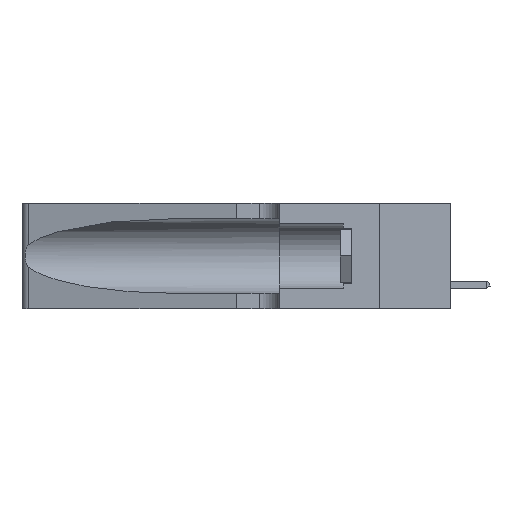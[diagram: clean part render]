
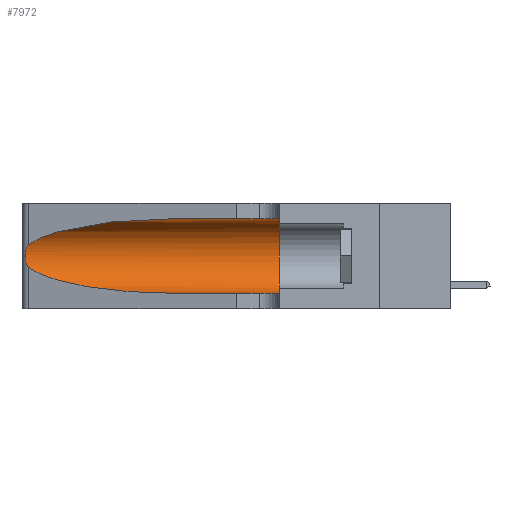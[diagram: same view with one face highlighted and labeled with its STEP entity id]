
A CAD part, left-side view. The second image highlights one B-rep face of the part: STEP entity #7972.
In plain terms, the highlighted cylindrical face has radius 3.308 mm (diameter 6.617 mm), a partial arc.
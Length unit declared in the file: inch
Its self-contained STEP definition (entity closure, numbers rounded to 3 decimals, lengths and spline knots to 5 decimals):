
#266 = CARTESIAN_POINT ( 'NONE',  ( 0.25555, 1.22993, 0.14849 ) ) ;
#973 = CARTESIAN_POINT ( 'NONE',  ( 0.1305, 0.72297, 0.05475 ) ) ;
#1196 = CARTESIAN_POINT ( 'NONE',  ( 0.25487, 1.22718, 0.14631 ) ) ;
#1910 = CARTESIAN_POINT ( 'NONE',  ( 0.1305, 0.35, 0.05475 ) ) ;
#3425 = CARTESIAN_POINT ( 'NONE',  ( 0.25555, 1.22994, 0.2215 ) ) ;
#3551 = CARTESIAN_POINT ( 'NONE',  ( 0.25487, 1.22718, 0.14631 ) ) ;
#4069 = DIRECTION ( 'NONE',  ( 0., 0., -1. ) ) ;
#4096 = EDGE_CURVE ( 'NONE', #28286, #34530, #33851, .T. ) ;
#5048 = VERTEX_POINT ( 'NONE', #1910 ) ;
#7972 = ADVANCED_FACE ( 'NONE', ( #28597 ), #37696, .F. ) ;
#8712 = CARTESIAN_POINT ( 'NONE',  ( 0.25487, 1.22718, 0.14631 ) ) ;
#9499 = ORIENTED_EDGE ( 'NONE', *, *, #19498, .T. ) ;
#9645 = CARTESIAN_POINT ( 'NONE',  ( 0.25487, 1.22718, 0.22369 ) ) ;
#9811 = CARTESIAN_POINT ( 'NONE',  ( 0.26018, 1.23835, 0.19895 ) ) ;
#9944 = CARTESIAN_POINT ( 'NONE',  ( 0.25639, 1.23184, 0.21858 ) ) ;
#10716 = CARTESIAN_POINT ( 'NONE',  ( 0.1305, 1.61858, 0.05475 ) ) ;
#10970 = VERTEX_POINT ( 'NONE', #23333 ) ;
#11529 = CARTESIAN_POINT ( 'NONE',  ( 0.1305, 0.72297, 0.05475 ) ) ;
#12513 = VERTEX_POINT ( 'NONE', #13545 ) ;
#13158 = CARTESIAN_POINT ( 'NONE',  ( 0.25789, 1.23486, 0.15765 ) ) ;
#13545 = CARTESIAN_POINT ( 'NONE',  ( 0.25487, 1.22718, 0.22369 ) ) ;
#16264 = CARTESIAN_POINT ( 'NONE',  ( 0.26075, 1.23896, 0.178 ) ) ;
#16585 = AXIS2_PLACEMENT_3D ( 'NONE', #17605, #33101, #27310 ) ;
#17440 = CARTESIAN_POINT ( 'NONE',  ( 0.2373, 1.15595, 0.08982 ) ) ;
#17605 = CARTESIAN_POINT ( 'NONE',  ( 0.1305, 0.35, 0.185 ) ) ;
#17712 = ORIENTED_EDGE ( 'NONE', *, *, #37765, .F. ) ;
#17723 = CARTESIAN_POINT ( 'NONE',  ( 0.18966, 0.96281, 0.05475 ) ) ;
#17938 = EDGE_LOOP ( 'NONE', ( #9499, #37967, #29278, #35419, #27481, #17712 ) ) ;
#19235 = CARTESIAN_POINT ( 'NONE',  ( 0.25854, 1.2359, 0.20912 ) ) ;
#19498 = EDGE_CURVE ( 'NONE', #28232, #12513, #19628, .T. ) ;
#19628 =( BOUNDED_CURVE ( )  B_SPLINE_CURVE ( 3, ( #27132, #28689, #23798, #9645 ),
 .UNSPECIFIED., .F., .F. ) 
 B_SPLINE_CURVE_WITH_KNOTS ( ( 4, 4 ),
 ( 1.5708, 2.84003 ),
 .UNSPECIFIED. ) 
 CURVE ( )  GEOMETRIC_REPRESENTATION_ITEM ( )  RATIONAL_B_SPLINE_CURVE ( ( 1., 0.87, 0.87, 1. ) ) 
 REPRESENTATION_ITEM ( '' )  );
#21260 = CARTESIAN_POINT ( 'NONE',  ( 0.1305, 0.72297, 0.31525 ) ) ;
#21829 = CIRCLE ( 'NONE', #16585, 0.13025 ) ;
#22750 = CARTESIAN_POINT ( 'NONE',  ( 0.25787, 1.23484, 0.2124 ) ) ;
#22917 = VECTOR ( 'NONE', #32781, 39.37008 ) ;
#23333 = CARTESIAN_POINT ( 'NONE',  ( 0.1305, 0.35, 0.31525 ) ) ;
#23798 = CARTESIAN_POINT ( 'NONE',  ( 0.2373, 1.15595, 0.28018 ) ) ;
#26509 = DIRECTION ( 'NONE',  ( 0., -1., 0. ) ) ;
#26532 = EDGE_CURVE ( 'NONE', #12513, #28286, #36415, .T. ) ;
#27076 = AXIS2_PLACEMENT_3D ( 'NONE', #28669, #26509, #4069 ) ;
#27132 = CARTESIAN_POINT ( 'NONE',  ( 0.1305, 0.72297, 0.31525 ) ) ;
#27310 = DIRECTION ( 'NONE',  ( 0., 0., 1. ) ) ;
#27481 = ORIENTED_EDGE ( 'NONE', *, *, #29092, .F. ) ;
#28232 = VERTEX_POINT ( 'NONE', #21260 ) ;
#28286 = VERTEX_POINT ( 'NONE', #8712 ) ;
#28597 = FACE_OUTER_BOUND ( 'NONE', #17938, .T. ) ;
#28669 = CARTESIAN_POINT ( 'NONE',  ( 0.1305, 1.61858, 0.185 ) ) ;
#28689 = CARTESIAN_POINT ( 'NONE',  ( 0.18966, 0.96281, 0.31525 ) ) ;
#28943 = CARTESIAN_POINT ( 'NONE',  ( 0.26075, 1.23896, 0.19203 ) ) ;
#29024 = VECTOR ( 'NONE', #39477, 39.37008 ) ;
#29092 = EDGE_CURVE ( 'NONE', #10970, #5048, #21829, .T. ) ;
#29209 = CARTESIAN_POINT ( 'NONE',  ( 0.26017, 1.23833, 0.17102 ) ) ;
#29278 = ORIENTED_EDGE ( 'NONE', *, *, #4096, .T. ) ;
#29430 = LINE ( 'NONE', #35769, #22917 ) ;
#32454 = CARTESIAN_POINT ( 'NONE',  ( 0.25856, 1.23593, 0.16098 ) ) ;
#32781 = DIRECTION ( 'NONE',  ( 0., -1., 0. ) ) ;
#33101 = DIRECTION ( 'NONE',  ( 0., 1., 0. ) ) ;
#33523 = LINE ( 'NONE', #10716, #29024 ) ;
#33851 =( BOUNDED_CURVE ( )  B_SPLINE_CURVE ( 3, ( #1196, #17440, #17723, #11529 ),
 .UNSPECIFIED., .F., .F. ) 
 B_SPLINE_CURVE_WITH_KNOTS ( ( 4, 4 ),
 ( 3.44316, 4.71239 ),
 .UNSPECIFIED. ) 
 CURVE ( )  GEOMETRIC_REPRESENTATION_ITEM ( )  RATIONAL_B_SPLINE_CURVE ( ( 1., 0.87, 0.87, 1. ) ) 
 REPRESENTATION_ITEM ( '' )  );
#34530 = VERTEX_POINT ( 'NONE', #973 ) ;
#35192 = CARTESIAN_POINT ( 'NONE',  ( 0.25487, 1.22718, 0.22369 ) ) ;
#35419 = ORIENTED_EDGE ( 'NONE', *, *, #37110, .T. ) ;
#35705 = CARTESIAN_POINT ( 'NONE',  ( 0.25639, 1.23186, 0.15144 ) ) ;
#35769 = CARTESIAN_POINT ( 'NONE',  ( 0.1305, 1.61858, 0.31525 ) ) ;
#36415 = B_SPLINE_CURVE_WITH_KNOTS ( 'NONE', 3,
 ( #35192, #3425, #9944, #22750, #19235, #9811, #28943, #16264, #29209, #32454, #13158, #35705, #266, #3551 ),
 .UNSPECIFIED., .F., .F.,
 ( 4, 2, 2, 2, 2, 2, 4 ),
 ( 0., 0.00027, 0.00053, 0.00107, 0.0016, 0.00187, 0.00214 ),
 .UNSPECIFIED. ) ;
#37110 = EDGE_CURVE ( 'NONE', #34530, #5048, #33523, .T. ) ;
#37696 = CYLINDRICAL_SURFACE ( 'NONE', #27076, 0.13025 ) ;
#37765 = EDGE_CURVE ( 'NONE', #28232, #10970, #29430, .T. ) ;
#37967 = ORIENTED_EDGE ( 'NONE', *, *, #26532, .T. ) ;
#39477 = DIRECTION ( 'NONE',  ( 0., -1., 0. ) ) ;
